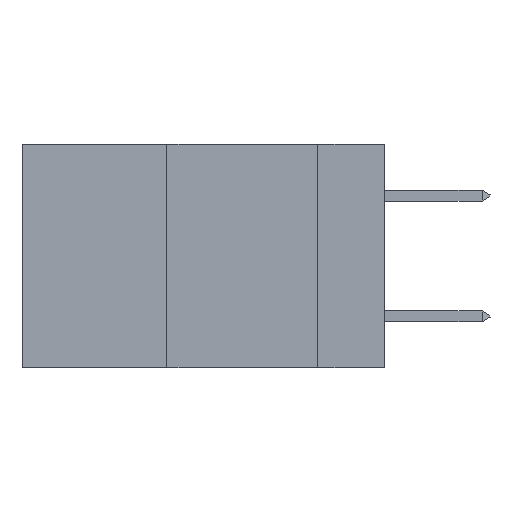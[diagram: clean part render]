
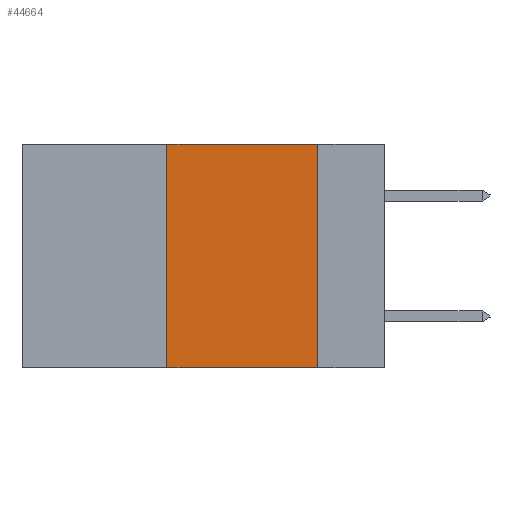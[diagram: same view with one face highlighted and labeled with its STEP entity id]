
A CAD part, left-side view. The second image highlights one B-rep face of the part: STEP entity #44664.
In plain terms, the highlighted planar face has unit normal (-1, 0, 0).
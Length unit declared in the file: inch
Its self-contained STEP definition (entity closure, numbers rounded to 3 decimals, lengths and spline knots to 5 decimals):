
#1351 = DIRECTION ( 'NONE',  ( 0., -1., 0. ) ) ;
#1699 = VECTOR ( 'NONE', #49543, 39.37008 ) ;
#3719 = PLANE ( 'NONE',  #42047 ) ;
#4231 = DIRECTION ( 'NONE',  ( 0., 0., -1. ) ) ;
#4863 = VECTOR ( 'NONE', #1351, 39.37008 ) ;
#6314 = CARTESIAN_POINT ( 'NONE',  ( 0., 0.36, 0. ) ) ;
#8440 = CARTESIAN_POINT ( 'NONE',  ( 0., 0.36, 0. ) ) ;
#10064 = EDGE_CURVE ( 'NONE', #19074, #14451, #22874, .T. ) ;
#11756 = ORIENTED_EDGE ( 'NONE', *, *, #10064, .F. ) ;
#12459 = CARTESIAN_POINT ( 'NONE',  ( 0., 0.11, 0. ) ) ;
#14066 = VECTOR ( 'NONE', #44790, 39.37008 ) ;
#14084 = ORIENTED_EDGE ( 'NONE', *, *, #29155, .F. ) ;
#14217 = DIRECTION ( 'NONE',  ( 0., 0., -1. ) ) ;
#14227 = ORIENTED_EDGE ( 'NONE', *, *, #34766, .T. ) ;
#14451 = VERTEX_POINT ( 'NONE', #12459 ) ;
#16052 = DIRECTION ( 'NONE',  ( 1., 0., 0. ) ) ;
#18247 = EDGE_LOOP ( 'NONE', ( #23897, #11756, #14084, #14227 ) ) ;
#19074 = VERTEX_POINT ( 'NONE', #6314 ) ;
#19618 = CARTESIAN_POINT ( 'NONE',  ( 0., 0.11, -0.37 ) ) ;
#21136 = VECTOR ( 'NONE', #14217, 39.37008 ) ;
#22874 = LINE ( 'NONE', #25464, #4863 ) ;
#23897 = ORIENTED_EDGE ( 'NONE', *, *, #38486, .F. ) ;
#25464 = CARTESIAN_POINT ( 'NONE',  ( 0., 0.6, 0. ) ) ;
#27000 = VERTEX_POINT ( 'NONE', #50244 ) ;
#29155 = EDGE_CURVE ( 'NONE', #27000, #19074, #38403, .T. ) ;
#29874 = CARTESIAN_POINT ( 'NONE',  ( 0., 0.11, 0. ) ) ;
#31727 = LINE ( 'NONE', #29874, #21136 ) ;
#33935 = CARTESIAN_POINT ( 'NONE',  ( 0., 0.6, -0.37 ) ) ;
#34669 = LINE ( 'NONE', #33935, #1699 ) ;
#34766 = EDGE_CURVE ( 'NONE', #27000, #50903, #34669, .T. ) ;
#38403 = LINE ( 'NONE', #8440, #14066 ) ;
#38486 = EDGE_CURVE ( 'NONE', #14451, #50903, #31727, .T. ) ;
#39860 = CARTESIAN_POINT ( 'NONE',  ( 0., 0.6, 0. ) ) ;
#40967 = FACE_OUTER_BOUND ( 'NONE', #18247, .T. ) ;
#42047 = AXIS2_PLACEMENT_3D ( 'NONE', #39860, #16052, #4231 ) ;
#44664 = ADVANCED_FACE ( 'NONE', ( #40967 ), #3719, .F. ) ;
#44790 = DIRECTION ( 'NONE',  ( 0., 0., 1. ) ) ;
#49543 = DIRECTION ( 'NONE',  ( 0., -1., 0. ) ) ;
#50244 = CARTESIAN_POINT ( 'NONE',  ( 0., 0.36, -0.37 ) ) ;
#50903 = VERTEX_POINT ( 'NONE', #19618 ) ;
